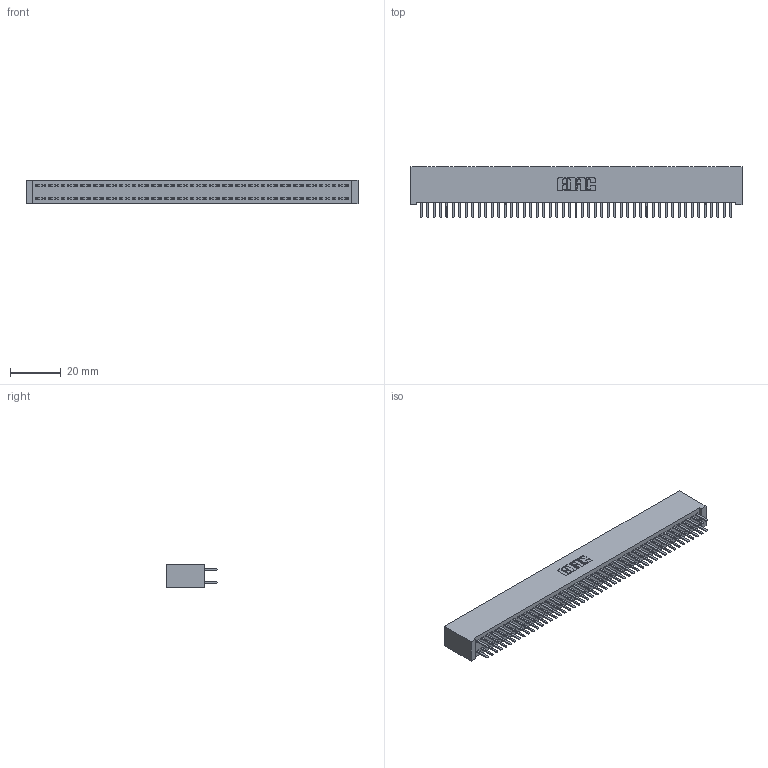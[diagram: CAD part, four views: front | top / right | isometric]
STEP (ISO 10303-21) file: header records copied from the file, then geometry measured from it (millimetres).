
FILE_DESCRIPTION (( 'STEP AP203' ), '1' );
FILE_NAME ('392-098-520-201.STEP', '2019-10-09T20:09:43', ( '' ), ( '' ), 'SwSTEP 2.0', 'SolidWorks 2016', '' );
FILE_SCHEMA (( 'CONFIG_CONTROL_DESIGN' ));
Length unit declared in the file: inch
Products named in the file (3): 342 Part_Lugless; 345-292-001_345-293-120; 392-098-520-201
Assembly tree (99 placements, depth 2):
  392-098-520-201
    342 Part_Lugless
    345-292-001_345-293-120  x98
Bounding box: 130.71 x 20.02 x 9.4 mm (x, y, z)
Volume: 12173.7 mm3; surface area: 20332.8 mm2
Topology: 99 solids, 99 shells, 5590 faces, 16249 edges, 10570 vertices
Faces by surface type: plane 3786, cylinder 1804
Entity records: 30323 total; most frequent: CARTESIAN_POINT 5026, ORIENTED_EDGE 4950, DIRECTION 4263, EDGE_CURVE 2475, VECTOR 2351, LINE 2351, VERTEX_POINT 1646, AXIS2_PLACEMENT_3D 956
